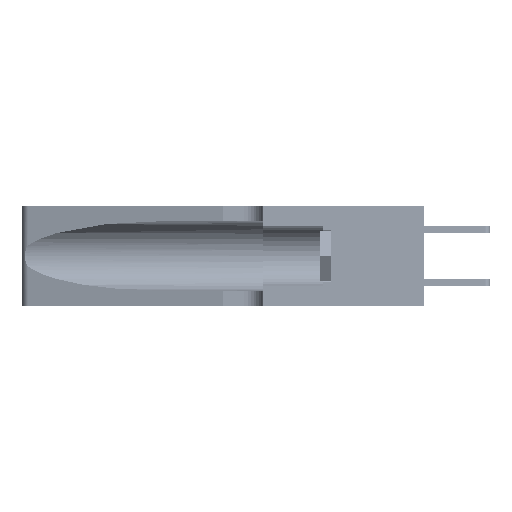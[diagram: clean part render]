
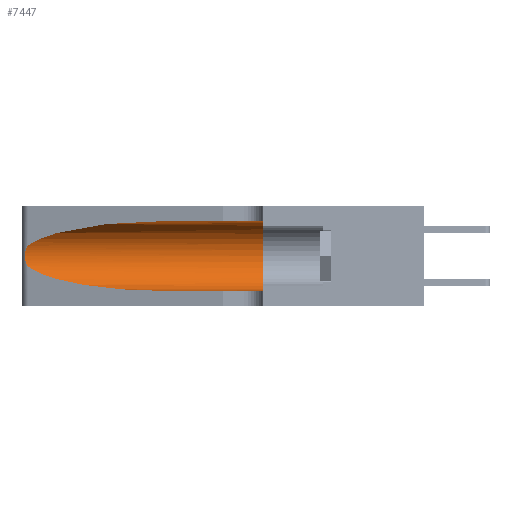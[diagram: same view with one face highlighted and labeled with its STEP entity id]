
A CAD part, left-side view. The second image highlights one B-rep face of the part: STEP entity #7447.
In plain terms, the highlighted cylindrical face has radius 3.308 mm (diameter 6.617 mm), a partial arc.
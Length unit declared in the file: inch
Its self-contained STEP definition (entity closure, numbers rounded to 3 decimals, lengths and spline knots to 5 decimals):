
#72 = CARTESIAN_POINT ( 'NONE',  ( 0.1305, 0.72297, 0.05475 ) ) ;
#292 =( BOUNDED_CURVE ( )  B_SPLINE_CURVE ( 3, ( #10428, #46756, #25072, #36446 ),
 .UNSPECIFIED., .F., .F. ) 
 B_SPLINE_CURVE_WITH_KNOTS ( ( 4, 4 ),
 ( 3.44316, 4.71239 ),
 .UNSPECIFIED. ) 
 CURVE ( )  GEOMETRIC_REPRESENTATION_ITEM ( )  RATIONAL_B_SPLINE_CURVE ( ( 1., 0.87, 0.87, 1. ) ) 
 REPRESENTATION_ITEM ( '' )  );
#1857 = CARTESIAN_POINT ( 'NONE',  ( 0.1305, 0.35, 0.05475 ) ) ;
#4638 = DIRECTION ( 'NONE',  ( 0., -1., 0. ) ) ;
#4695 = CARTESIAN_POINT ( 'NONE',  ( 0.1305, 0.35, 0.185 ) ) ;
#4754 = EDGE_CURVE ( 'NONE', #34909, #33609, #5860, .T. ) ;
#5860 = LINE ( 'NONE', #36578, #14899 ) ;
#7447 = ADVANCED_FACE ( 'NONE', ( #45801 ), #9061, .F. ) ;
#7724 = DIRECTION ( 'NONE',  ( 0., -1., 0. ) ) ;
#9061 = CYLINDRICAL_SURFACE ( 'NONE', #24262, 0.13025 ) ;
#9441 = AXIS2_PLACEMENT_3D ( 'NONE', #4695, #29931, #18873 ) ;
#9513 = VERTEX_POINT ( 'NONE', #15188 ) ;
#10428 = CARTESIAN_POINT ( 'NONE',  ( 0.25487, 1.22718, 0.14631 ) ) ;
#11786 = ORIENTED_EDGE ( 'NONE', *, *, #39435, .T. ) ;
#12259 = EDGE_LOOP ( 'NONE', ( #19579, #11786, #39561, #41587, #39204, #38736 ) ) ;
#12514 = VERTEX_POINT ( 'NONE', #22066 ) ;
#12642 = VERTEX_POINT ( 'NONE', #30615 ) ;
#12999 = CARTESIAN_POINT ( 'NONE',  ( 0.25487, 1.22718, 0.22369 ) ) ;
#13057 = EDGE_CURVE ( 'NONE', #41083, #12514, #23889, .T. ) ;
#13274 = CARTESIAN_POINT ( 'NONE',  ( 0.1305, 0.72297, 0.31525 ) ) ;
#13564 = B_SPLINE_CURVE_WITH_KNOTS ( 'NONE', 3,
 ( #12999, #45394, #41595, #34447, #34608, #30686, #19920, #38088, #45230, #16002, #16460, #23876, #19631, #23711 ),
 .UNSPECIFIED., .F., .F.,
 ( 4, 2, 2, 2, 2, 2, 4 ),
 ( 0., 0.00027, 0.00053, 0.00107, 0.0016, 0.00187, 0.00214 ),
 .UNSPECIFIED. ) ;
#14899 = VECTOR ( 'NONE', #18263, 39.37008 ) ;
#15188 = CARTESIAN_POINT ( 'NONE',  ( 0.25487, 1.22718, 0.22369 ) ) ;
#16002 = CARTESIAN_POINT ( 'NONE',  ( 0.25856, 1.23593, 0.16098 ) ) ;
#16460 = CARTESIAN_POINT ( 'NONE',  ( 0.25789, 1.23486, 0.15765 ) ) ;
#16576 = CARTESIAN_POINT ( 'NONE',  ( 0.1305, 0.72297, 0.31525 ) ) ;
#17881 = EDGE_CURVE ( 'NONE', #41083, #9513, #25839, .T. ) ;
#18263 = DIRECTION ( 'NONE',  ( 0., -1., 0. ) ) ;
#18873 = DIRECTION ( 'NONE',  ( 0., 0., 1. ) ) ;
#19579 = ORIENTED_EDGE ( 'NONE', *, *, #17881, .T. ) ;
#19631 = CARTESIAN_POINT ( 'NONE',  ( 0.25555, 1.22993, 0.14849 ) ) ;
#19680 = EDGE_CURVE ( 'NONE', #12642, #34909, #292, .T. ) ;
#19920 = CARTESIAN_POINT ( 'NONE',  ( 0.26075, 1.23896, 0.19203 ) ) ;
#21701 = CARTESIAN_POINT ( 'NONE',  ( 0.25487, 1.22718, 0.22369 ) ) ;
#22066 = CARTESIAN_POINT ( 'NONE',  ( 0.1305, 0.35, 0.31525 ) ) ;
#23711 = CARTESIAN_POINT ( 'NONE',  ( 0.25487, 1.22718, 0.14631 ) ) ;
#23876 = CARTESIAN_POINT ( 'NONE',  ( 0.25639, 1.23186, 0.15144 ) ) ;
#23889 = LINE ( 'NONE', #25196, #24480 ) ;
#24262 = AXIS2_PLACEMENT_3D ( 'NONE', #37264, #4638, #26073 ) ;
#24480 = VECTOR ( 'NONE', #7724, 39.37008 ) ;
#24783 = CIRCLE ( 'NONE', #9441, 0.13025 ) ;
#25072 = CARTESIAN_POINT ( 'NONE',  ( 0.18966, 0.96281, 0.05475 ) ) ;
#25196 = CARTESIAN_POINT ( 'NONE',  ( 0.1305, 1.61858, 0.31525 ) ) ;
#25677 = CARTESIAN_POINT ( 'NONE',  ( 0.18966, 0.96281, 0.31525 ) ) ;
#25839 =( BOUNDED_CURVE ( )  B_SPLINE_CURVE ( 3, ( #13274, #25677, #43540, #21701 ),
 .UNSPECIFIED., .F., .T. ) 
 B_SPLINE_CURVE_WITH_KNOTS ( ( 4, 4 ),
 ( 1.5708, 2.84003 ),
 .UNSPECIFIED. ) 
 CURVE ( )  GEOMETRIC_REPRESENTATION_ITEM ( )  RATIONAL_B_SPLINE_CURVE ( ( 1., 0.87, 0.87, 1. ) ) 
 REPRESENTATION_ITEM ( '' )  );
#26073 = DIRECTION ( 'NONE',  ( 0., 0., -1. ) ) ;
#29931 = DIRECTION ( 'NONE',  ( 0., 1., 0. ) ) ;
#30615 = CARTESIAN_POINT ( 'NONE',  ( 0.25487, 1.22718, 0.14631 ) ) ;
#30686 = CARTESIAN_POINT ( 'NONE',  ( 0.26018, 1.23835, 0.19895 ) ) ;
#33609 = VERTEX_POINT ( 'NONE', #1857 ) ;
#34447 = CARTESIAN_POINT ( 'NONE',  ( 0.25787, 1.23484, 0.2124 ) ) ;
#34608 = CARTESIAN_POINT ( 'NONE',  ( 0.25854, 1.2359, 0.20912 ) ) ;
#34909 = VERTEX_POINT ( 'NONE', #72 ) ;
#36446 = CARTESIAN_POINT ( 'NONE',  ( 0.1305, 0.72297, 0.05475 ) ) ;
#36578 = CARTESIAN_POINT ( 'NONE',  ( 0.1305, 1.61858, 0.05475 ) ) ;
#37264 = CARTESIAN_POINT ( 'NONE',  ( 0.1305, 1.61858, 0.185 ) ) ;
#38088 = CARTESIAN_POINT ( 'NONE',  ( 0.26075, 1.23896, 0.178 ) ) ;
#38736 = ORIENTED_EDGE ( 'NONE', *, *, #13057, .F. ) ;
#39204 = ORIENTED_EDGE ( 'NONE', *, *, #42248, .F. ) ;
#39435 = EDGE_CURVE ( 'NONE', #9513, #12642, #13564, .T. ) ;
#39561 = ORIENTED_EDGE ( 'NONE', *, *, #19680, .T. ) ;
#41083 = VERTEX_POINT ( 'NONE', #16576 ) ;
#41587 = ORIENTED_EDGE ( 'NONE', *, *, #4754, .T. ) ;
#41595 = CARTESIAN_POINT ( 'NONE',  ( 0.25639, 1.23184, 0.21858 ) ) ;
#42248 = EDGE_CURVE ( 'NONE', #12514, #33609, #24783, .T. ) ;
#43540 = CARTESIAN_POINT ( 'NONE',  ( 0.2373, 1.15595, 0.28018 ) ) ;
#45230 = CARTESIAN_POINT ( 'NONE',  ( 0.26017, 1.23833, 0.17102 ) ) ;
#45394 = CARTESIAN_POINT ( 'NONE',  ( 0.25555, 1.22994, 0.2215 ) ) ;
#45801 = FACE_OUTER_BOUND ( 'NONE', #12259, .T. ) ;
#46756 = CARTESIAN_POINT ( 'NONE',  ( 0.2373, 1.15595, 0.08982 ) ) ;
